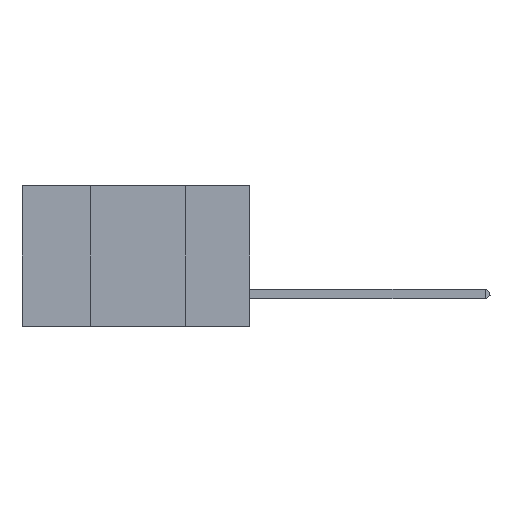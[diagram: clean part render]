
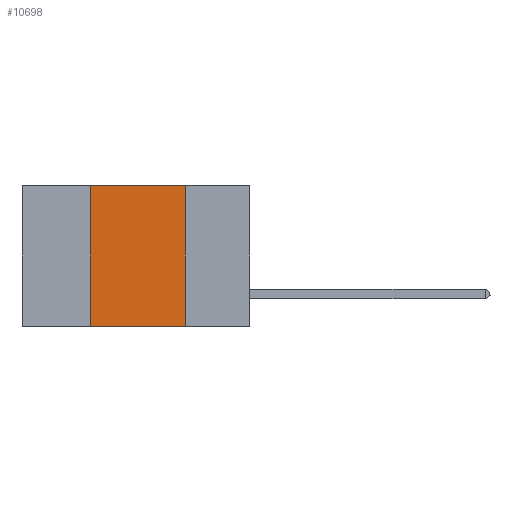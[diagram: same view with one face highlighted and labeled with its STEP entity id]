
A CAD part, left-side view. The second image highlights one B-rep face of the part: STEP entity #10698.
In plain terms, the highlighted planar face has unit normal (-1, 0, 0).
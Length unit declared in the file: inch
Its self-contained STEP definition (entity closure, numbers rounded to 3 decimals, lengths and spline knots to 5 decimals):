
#928 = LINE ( 'NONE', #22340, #3717 ) ;
#1248 = VECTOR ( 'NONE', #15380, 39.37008 ) ;
#1979 = VERTEX_POINT ( 'NONE', #3764 ) ;
#2872 = CARTESIAN_POINT ( 'NONE',  ( 0., 0.42, 0. ) ) ;
#3711 = CARTESIAN_POINT ( 'NONE',  ( 0., 0.42, -0.37 ) ) ;
#3717 = VECTOR ( 'NONE', #13451, 39.37008 ) ;
#3764 = CARTESIAN_POINT ( 'NONE',  ( 0., 0.17, -0.37 ) ) ;
#3774 = CARTESIAN_POINT ( 'NONE',  ( 0., 0.17, 0. ) ) ;
#4598 = EDGE_CURVE ( 'NONE', #10983, #22393, #21704, .T. ) ;
#4622 = DIRECTION ( 'NONE',  ( 0., 0., -1. ) ) ;
#4746 = AXIS2_PLACEMENT_3D ( 'NONE', #15273, #13547, #4622 ) ;
#4837 = LINE ( 'NONE', #2872, #1248 ) ;
#5038 = VERTEX_POINT ( 'NONE', #3711 ) ;
#5587 = DIRECTION ( 'NONE',  ( 0., 0., -1. ) ) ;
#9651 = ORIENTED_EDGE ( 'NONE', *, *, #19150, .T. ) ;
#10506 = EDGE_LOOP ( 'NONE', ( #16595, #20318, #20874, #9651 ) ) ;
#10698 = ADVANCED_FACE ( 'NONE', ( #17850 ), #15580, .F. ) ;
#10825 = CARTESIAN_POINT ( 'NONE',  ( 0., 0.17, 0. ) ) ;
#10983 = VERTEX_POINT ( 'NONE', #18458 ) ;
#12796 = CARTESIAN_POINT ( 'NONE',  ( 0., 0.6, 0. ) ) ;
#13451 = DIRECTION ( 'NONE',  ( 0., -1., 0. ) ) ;
#13547 = DIRECTION ( 'NONE',  ( 1., 0., 0. ) ) ;
#15273 = CARTESIAN_POINT ( 'NONE',  ( 0., 0.6, 0. ) ) ;
#15380 = DIRECTION ( 'NONE',  ( 0., 0., 1. ) ) ;
#15580 = PLANE ( 'NONE',  #4746 ) ;
#16595 = ORIENTED_EDGE ( 'NONE', *, *, #23041, .F. ) ;
#17850 = FACE_OUTER_BOUND ( 'NONE', #10506, .T. ) ;
#18180 = EDGE_CURVE ( 'NONE', #5038, #10983, #4837, .T. ) ;
#18458 = CARTESIAN_POINT ( 'NONE',  ( 0., 0.42, 0. ) ) ;
#19150 = EDGE_CURVE ( 'NONE', #5038, #1979, #928, .T. ) ;
#19374 = VECTOR ( 'NONE', #5587, 39.37008 ) ;
#19926 = LINE ( 'NONE', #3774, #19374 ) ;
#20318 = ORIENTED_EDGE ( 'NONE', *, *, #4598, .F. ) ;
#20874 = ORIENTED_EDGE ( 'NONE', *, *, #18180, .F. ) ;
#21147 = VECTOR ( 'NONE', #21627, 39.37008 ) ;
#21627 = DIRECTION ( 'NONE',  ( 0., -1., 0. ) ) ;
#21704 = LINE ( 'NONE', #12796, #21147 ) ;
#22340 = CARTESIAN_POINT ( 'NONE',  ( 0., 0.6, -0.37 ) ) ;
#22393 = VERTEX_POINT ( 'NONE', #10825 ) ;
#23041 = EDGE_CURVE ( 'NONE', #22393, #1979, #19926, .T. ) ;
